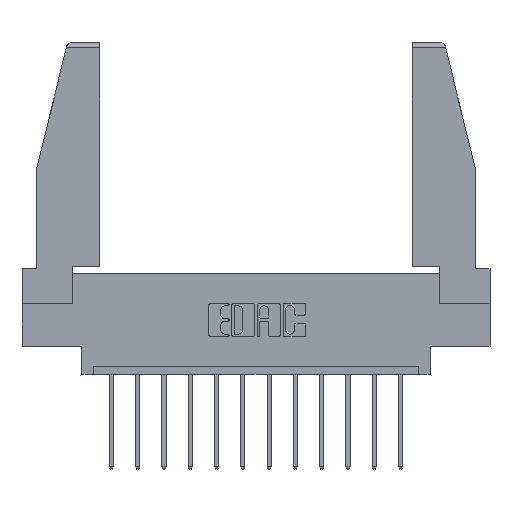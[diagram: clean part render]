
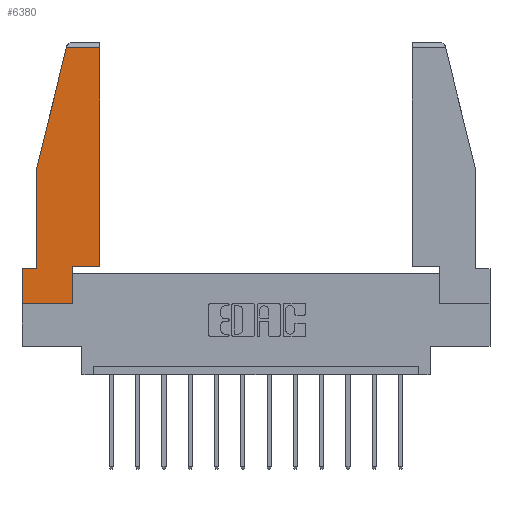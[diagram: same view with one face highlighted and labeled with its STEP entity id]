
A CAD part, top view. The second image highlights one B-rep face of the part: STEP entity #6380.
In plain terms, the highlighted planar face has unit normal (0, 0, 1).
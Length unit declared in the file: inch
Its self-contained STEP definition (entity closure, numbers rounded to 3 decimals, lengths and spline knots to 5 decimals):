
#88 = VECTOR ( 'NONE', #760, 39.37008 ) ;
#273 = DIRECTION ( 'NONE',  ( 0., 1., 0. ) ) ;
#603 = CARTESIAN_POINT ( 'NONE',  ( 0.086, 0.8, 0. ) ) ;
#711 = LINE ( 'NONE', #7329, #14102 ) ;
#760 = DIRECTION ( 'NONE',  ( 1., 0., 0. ) ) ;
#925 = DIRECTION ( 'NONE',  ( -1., 0., 0. ) ) ;
#1330 = DIRECTION ( 'NONE',  ( 0., -1., 0. ) ) ;
#1539 = ORIENTED_EDGE ( 'NONE', *, *, #15014, .T. ) ;
#1627 = CARTESIAN_POINT ( 'NONE',  ( 0.297, 0., 0. ) ) ;
#1678 = DIRECTION ( 'NONE',  ( -0.239, -0.971, 0. ) ) ;
#2219 = CARTESIAN_POINT ( 'NONE',  ( 0.461, 0.223, 0. ) ) ;
#2272 = LINE ( 'NONE', #11740, #11381 ) ;
#2315 = CARTESIAN_POINT ( 'NONE',  ( 0., 0., 0. ) ) ;
#2321 = EDGE_CURVE ( 'NONE', #3001, #11384, #4673, .T. ) ;
#2438 = EDGE_CURVE ( 'NONE', #2542, #13484, #9006, .T. ) ;
#2502 = CARTESIAN_POINT ( 'NONE',  ( 0.297, 0.223, 0. ) ) ;
#2542 = VERTEX_POINT ( 'NONE', #1627 ) ;
#2688 = VECTOR ( 'NONE', #273, 39.37008 ) ;
#2785 = CARTESIAN_POINT ( 'NONE',  ( 0., 0., 0. ) ) ;
#3001 = VERTEX_POINT ( 'NONE', #10228 ) ;
#3237 = LINE ( 'NONE', #12637, #88 ) ;
#3786 = CARTESIAN_POINT ( 'NONE',  ( 0.271, 1.55, 0. ) ) ;
#4535 = EDGE_CURVE ( 'NONE', #10648, #7443, #6334, .T. ) ;
#4673 = LINE ( 'NONE', #603, #8636 ) ;
#4943 = VECTOR ( 'NONE', #1678, 39.37008 ) ;
#4970 = CARTESIAN_POINT ( 'NONE',  ( 0., 0., 0. ) ) ;
#4998 = CARTESIAN_POINT ( 'NONE',  ( 0.297, 0., 0. ) ) ;
#5427 = AXIS2_PLACEMENT_3D ( 'NONE', #4970, #13294, #9762 ) ;
#5872 = CARTESIAN_POINT ( 'NONE',  ( 0., 0.21, 0. ) ) ;
#6118 = EDGE_LOOP ( 'NONE', ( #9705, #6229, #12314, #6827, #14783, #13238, #8351, #14235, #1539 ) ) ;
#6229 = ORIENTED_EDGE ( 'NONE', *, *, #6284, .T. ) ;
#6284 = EDGE_CURVE ( 'NONE', #7443, #11720, #11295, .T. ) ;
#6317 = DIRECTION ( 'NONE',  ( 1., 0., 0. ) ) ;
#6334 = LINE ( 'NONE', #8184, #11914 ) ;
#6380 = ADVANCED_FACE ( 'NONE', ( #6455 ), #13399, .T. ) ;
#6455 = FACE_OUTER_BOUND ( 'NONE', #6118, .T. ) ;
#6617 = LINE ( 'NONE', #3786, #4943 ) ;
#6827 = ORIENTED_EDGE ( 'NONE', *, *, #2321, .T. ) ;
#7329 = CARTESIAN_POINT ( 'NONE',  ( 0., 0.21, 0. ) ) ;
#7443 = VERTEX_POINT ( 'NONE', #13127 ) ;
#7629 = VECTOR ( 'NONE', #6317, 39.37008 ) ;
#7826 = EDGE_CURVE ( 'NONE', #11720, #3001, #6617, .T. ) ;
#8184 = CARTESIAN_POINT ( 'NONE',  ( 0.461, 0.223, 0. ) ) ;
#8351 = ORIENTED_EDGE ( 'NONE', *, *, #11923, .T. ) ;
#8636 = VECTOR ( 'NONE', #12465, 39.37008 ) ;
#8908 = VERTEX_POINT ( 'NONE', #2315 ) ;
#9006 = LINE ( 'NONE', #4998, #2688 ) ;
#9705 = ORIENTED_EDGE ( 'NONE', *, *, #4535, .T. ) ;
#9762 = DIRECTION ( 'NONE',  ( 1., 0., 0. ) ) ;
#9819 = DIRECTION ( 'NONE',  ( -1., 0., 0. ) ) ;
#10214 = EDGE_CURVE ( 'NONE', #11384, #14393, #2272, .T. ) ;
#10228 = CARTESIAN_POINT ( 'NONE',  ( 0.086, 0.8, 0. ) ) ;
#10648 = VERTEX_POINT ( 'NONE', #2219 ) ;
#10660 = DIRECTION ( 'NONE',  ( 0., 1., 0. ) ) ;
#11257 = CARTESIAN_POINT ( 'NONE',  ( 0.2636, 1.52, 0. ) ) ;
#11295 = LINE ( 'NONE', #14496, #13701 ) ;
#11381 = VECTOR ( 'NONE', #925, 39.37008 ) ;
#11384 = VERTEX_POINT ( 'NONE', #14082 ) ;
#11720 = VERTEX_POINT ( 'NONE', #11257 ) ;
#11740 = CARTESIAN_POINT ( 'NONE',  ( 0., 0.21, 0. ) ) ;
#11914 = VECTOR ( 'NONE', #10660, 39.37008 ) ;
#11923 = EDGE_CURVE ( 'NONE', #8908, #2542, #14317, .T. ) ;
#12314 = ORIENTED_EDGE ( 'NONE', *, *, #7826, .T. ) ;
#12465 = DIRECTION ( 'NONE',  ( 0., -1., 0. ) ) ;
#12637 = CARTESIAN_POINT ( 'NONE',  ( 0.297, 0.223, 0. ) ) ;
#13127 = CARTESIAN_POINT ( 'NONE',  ( 0.461, 1.52, 0. ) ) ;
#13238 = ORIENTED_EDGE ( 'NONE', *, *, #13618, .T. ) ;
#13294 = DIRECTION ( 'NONE',  ( 0., 0., 1. ) ) ;
#13399 = PLANE ( 'NONE',  #5427 ) ;
#13484 = VERTEX_POINT ( 'NONE', #2502 ) ;
#13618 = EDGE_CURVE ( 'NONE', #14393, #8908, #711, .T. ) ;
#13701 = VECTOR ( 'NONE', #9819, 39.37008 ) ;
#14082 = CARTESIAN_POINT ( 'NONE',  ( 0.086, 0.21, 0. ) ) ;
#14102 = VECTOR ( 'NONE', #1330, 39.37008 ) ;
#14235 = ORIENTED_EDGE ( 'NONE', *, *, #2438, .T. ) ;
#14317 = LINE ( 'NONE', #2785, #7629 ) ;
#14393 = VERTEX_POINT ( 'NONE', #5872 ) ;
#14496 = CARTESIAN_POINT ( 'NONE',  ( 0., 1.52, 0. ) ) ;
#14783 = ORIENTED_EDGE ( 'NONE', *, *, #10214, .T. ) ;
#15014 = EDGE_CURVE ( 'NONE', #13484, #10648, #3237, .T. ) ;
